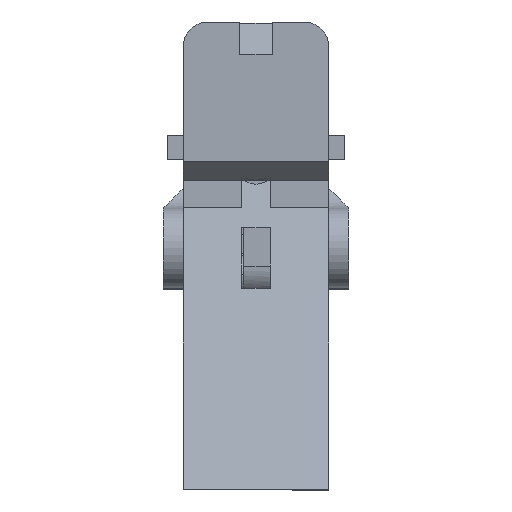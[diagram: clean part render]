
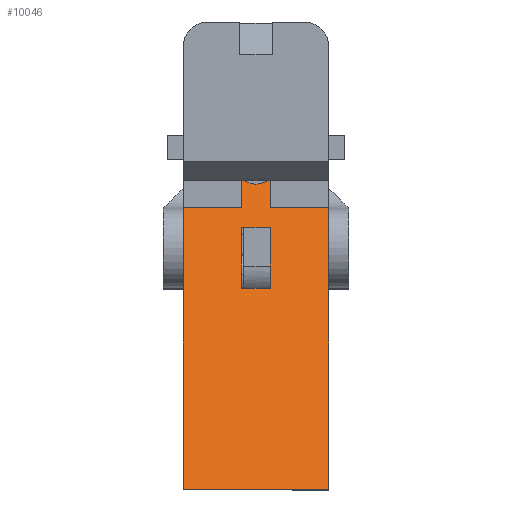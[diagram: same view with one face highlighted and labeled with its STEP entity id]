
A CAD part, top view. The second image highlights one B-rep face of the part: STEP entity #10046.
In plain terms, the highlighted face is planar.
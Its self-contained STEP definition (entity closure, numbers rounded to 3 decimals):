
#86 = LINE ( 'NONE', #7831, #7262 ) ;
#330 = AXIS2_PLACEMENT_3D ( 'NONE', #9895, #2735, #12780 ) ;
#509 = VERTEX_POINT ( 'NONE', #10830 ) ;
#756 = DIRECTION ( 'NONE',  ( 0., 0., -1. ) ) ;
#983 = CARTESIAN_POINT ( 'NONE',  ( -52.728, -42.47, 10.75 ) ) ;
#1105 = ORIENTED_EDGE ( 'NONE', *, *, #10426, .T. ) ;
#1141 = CARTESIAN_POINT ( 'NONE',  ( -43.64, -17.5, 0. ) ) ;
#1212 = DIRECTION ( 'NONE',  ( -0.342, -0.94, 0. ) ) ;
#1278 = PLANE ( 'NONE',  #330 ) ;
#1321 = DIRECTION ( 'NONE',  ( 0., 0., -1. ) ) ;
#1440 = CARTESIAN_POINT ( 'NONE',  ( -40.91, -10., 0. ) ) ;
#1559 = EDGE_CURVE ( 'NONE', #14070, #5068, #11446, .T. ) ;
#1646 = FACE_BOUND ( 'NONE', #4296, .T. ) ;
#1700 = CARTESIAN_POINT ( 'NONE',  ( -40.91, -10., 3.5 ) ) ;
#2232 = EDGE_CURVE ( 'NONE', #5544, #7264, #13898, .T. ) ;
#2548 = ORIENTED_EDGE ( 'NONE', *, *, #17016, .F. ) ;
#2624 = ORIENTED_EDGE ( 'NONE', *, *, #13725, .F. ) ;
#2672 = EDGE_CURVE ( 'NONE', #509, #7773, #9855, .T. ) ;
#2735 = DIRECTION ( 'NONE',  ( -0.94, 0.342, 0. ) ) ;
#2800 = LINE ( 'NONE', #9377, #7072 ) ;
#3864 = DIRECTION ( 'NONE',  ( -0.342, -0.94, 0. ) ) ;
#4062 = EDGE_CURVE ( 'NONE', #15540, #14419, #10807, .T. ) ;
#4083 = CARTESIAN_POINT ( 'NONE',  ( -47.279, -27.5, -7.25 ) ) ;
#4296 = EDGE_LOOP ( 'NONE', ( #2548, #17075, #11305, #13177 ) ) ;
#4394 = CARTESIAN_POINT ( 'NONE',  ( -38.68, -3.873, 0. ) ) ;
#4594 = VECTOR ( 'NONE', #9723, 1000. ) ;
#5016 = FACE_OUTER_BOUND ( 'NONE', #15195, .T. ) ;
#5068 = VERTEX_POINT ( 'NONE', #1141 ) ;
#5478 = CARTESIAN_POINT ( 'NONE',  ( -47.279, -27.5, 3.5 ) ) ;
#5544 = VERTEX_POINT ( 'NONE', #9379 ) ;
#5860 = LINE ( 'NONE', #4083, #13516 ) ;
#6514 = CARTESIAN_POINT ( 'NONE',  ( -32.91, 11.978, 0. ) ) ;
#6839 = VECTOR ( 'NONE', #7666, 1000. ) ;
#6970 = CARTESIAN_POINT ( 'NONE',  ( -43.64, -17.5, 3.5 ) ) ;
#7036 = VERTEX_POINT ( 'NONE', #13040 ) ;
#7072 = VECTOR ( 'NONE', #756, 1000. ) ;
#7129 = ORIENTED_EDGE ( 'NONE', *, *, #13996, .F. ) ;
#7133 = VECTOR ( 'NONE', #1321, 1000. ) ;
#7262 = VECTOR ( 'NONE', #10704, 1000. ) ;
#7264 = VERTEX_POINT ( 'NONE', #12386 ) ;
#7302 = CARTESIAN_POINT ( 'NONE',  ( -39.053, -4.898, 2.475 ) ) ;
#7386 = EDGE_CURVE ( 'NONE', #509, #14884, #14326, .T. ) ;
#7666 = DIRECTION ( 'NONE',  ( 0., 0., 1. ) ) ;
#7773 = VERTEX_POINT ( 'NONE', #8422 ) ;
#7799 = ORIENTED_EDGE ( 'NONE', *, *, #7386, .T. ) ;
#7831 = CARTESIAN_POINT ( 'NONE',  ( -32.91, 11.978, 3.5 ) ) ;
#7849 =( BOUNDED_CURVE ( )  B_SPLINE_CURVE ( 3, ( #4394, #15874, #7302, #17296 ),
 .UNSPECIFIED., .F., .F. ) 
 B_SPLINE_CURVE_WITH_KNOTS ( ( 4, 4 ),
 ( 2.356, 3.927 ),
 .UNSPECIFIED. ) 
 CURVE ( )  GEOMETRIC_REPRESENTATION_ITEM ( )  RATIONAL_B_SPLINE_CURVE ( ( 1., 0.805, 0.805, 1. ) ) 
 REPRESENTATION_ITEM ( '' )  );
#8279 = CARTESIAN_POINT ( 'NONE',  ( -47.279, -27.5, 10.75 ) ) ;
#8422 = CARTESIAN_POINT ( 'NONE',  ( -38.68, -3.873, 0. ) ) ;
#8499 = DIRECTION ( 'NONE',  ( 0.342, 0.94, 0. ) ) ;
#8715 = ORIENTED_EDGE ( 'NONE', *, *, #2232, .F. ) ;
#8869 = EDGE_CURVE ( 'NONE', #5544, #15067, #16028, .T. ) ;
#9377 = CARTESIAN_POINT ( 'NONE',  ( -40.91, -10., 10.75 ) ) ;
#9379 = CARTESIAN_POINT ( 'NONE',  ( -52.728, -42.47, 10.75 ) ) ;
#9649 = CARTESIAN_POINT ( 'NONE',  ( -40., -7.5, -7.25 ) ) ;
#9723 = DIRECTION ( 'NONE',  ( 0.342, 0.94, 0. ) ) ;
#9855 = LINE ( 'NONE', #6514, #16094 ) ;
#9895 = CARTESIAN_POINT ( 'NONE',  ( -47.279, -27.5, 10.75 ) ) ;
#10046 = ADVANCED_FACE ( 'NONE', ( #5016, #1646 ), #1278, .T. ) ;
#10082 = VECTOR ( 'NONE', #16783, 1000. ) ;
#10426 = EDGE_CURVE ( 'NONE', #17170, #7036, #86, .T. ) ;
#10656 = LINE ( 'NONE', #18398, #6839 ) ;
#10704 = DIRECTION ( 'NONE',  ( 0.342, 0.94, 0. ) ) ;
#10807 = LINE ( 'NONE', #5478, #17950 ) ;
#10830 = CARTESIAN_POINT ( 'NONE',  ( -40., -7.5, 0. ) ) ;
#11305 = ORIENTED_EDGE ( 'NONE', *, *, #11676, .F. ) ;
#11397 = CARTESIAN_POINT ( 'NONE',  ( -40., -7.5, 10.75 ) ) ;
#11446 = LINE ( 'NONE', #12519, #15231 ) ;
#11613 = ORIENTED_EDGE ( 'NONE', *, *, #2672, .F. ) ;
#11676 = EDGE_CURVE ( 'NONE', #5068, #14419, #10656, .T. ) ;
#12219 = DIRECTION ( 'NONE',  ( 0.342, 0.94, 0. ) ) ;
#12324 = CARTESIAN_POINT ( 'NONE',  ( -40., -7.5, 10.75 ) ) ;
#12386 = CARTESIAN_POINT ( 'NONE',  ( -52.728, -42.47, -7.25 ) ) ;
#12519 = CARTESIAN_POINT ( 'NONE',  ( -47.279, -27.5, 0. ) ) ;
#12780 = DIRECTION ( 'NONE',  ( -0.342, -0.94, 0. ) ) ;
#13040 = CARTESIAN_POINT ( 'NONE',  ( -38.68, -3.873, 3.5 ) ) ;
#13177 = ORIENTED_EDGE ( 'NONE', *, *, #1559, .F. ) ;
#13383 = VECTOR ( 'NONE', #17063, 1000. ) ;
#13502 = ORIENTED_EDGE ( 'NONE', *, *, #8869, .T. ) ;
#13516 = VECTOR ( 'NONE', #8499, 1000. ) ;
#13725 = EDGE_CURVE ( 'NONE', #7773, #7036, #7849, .T. ) ;
#13898 = LINE ( 'NONE', #983, #10082 ) ;
#13965 = ORIENTED_EDGE ( 'NONE', *, *, #16403, .T. ) ;
#13996 = EDGE_CURVE ( 'NONE', #7264, #14884, #5860, .T. ) ;
#14070 = VERTEX_POINT ( 'NONE', #1440 ) ;
#14326 = LINE ( 'NONE', #11397, #7133 ) ;
#14419 = VERTEX_POINT ( 'NONE', #6970 ) ;
#14884 = VERTEX_POINT ( 'NONE', #9649 ) ;
#15067 = VERTEX_POINT ( 'NONE', #12324 ) ;
#15195 = EDGE_LOOP ( 'NONE', ( #2624, #11613, #7799, #7129, #8715, #13502, #13965, #1105 ) ) ;
#15231 = VECTOR ( 'NONE', #3864, 1000. ) ;
#15425 = CARTESIAN_POINT ( 'NONE',  ( -40., -7.5, 3.5 ) ) ;
#15540 = VERTEX_POINT ( 'NONE', #1700 ) ;
#15646 = CARTESIAN_POINT ( 'NONE',  ( -40., -7.5, 10.75 ) ) ;
#15874 = CARTESIAN_POINT ( 'NONE',  ( -39.053, -4.898, 1.025 ) ) ;
#16028 = LINE ( 'NONE', #8279, #4594 ) ;
#16094 = VECTOR ( 'NONE', #12219, 1000. ) ;
#16403 = EDGE_CURVE ( 'NONE', #15067, #17170, #17152, .T. ) ;
#16783 = DIRECTION ( 'NONE',  ( 0., 0., -1. ) ) ;
#17016 = EDGE_CURVE ( 'NONE', #15540, #14070, #2800, .T. ) ;
#17063 = DIRECTION ( 'NONE',  ( 0., 0., -1. ) ) ;
#17075 = ORIENTED_EDGE ( 'NONE', *, *, #4062, .T. ) ;
#17152 = LINE ( 'NONE', #15646, #13383 ) ;
#17170 = VERTEX_POINT ( 'NONE', #15425 ) ;
#17296 = CARTESIAN_POINT ( 'NONE',  ( -38.68, -3.873, 3.5 ) ) ;
#17950 = VECTOR ( 'NONE', #1212, 1000. ) ;
#18398 = CARTESIAN_POINT ( 'NONE',  ( -43.64, -17.5, 10.75 ) ) ;
